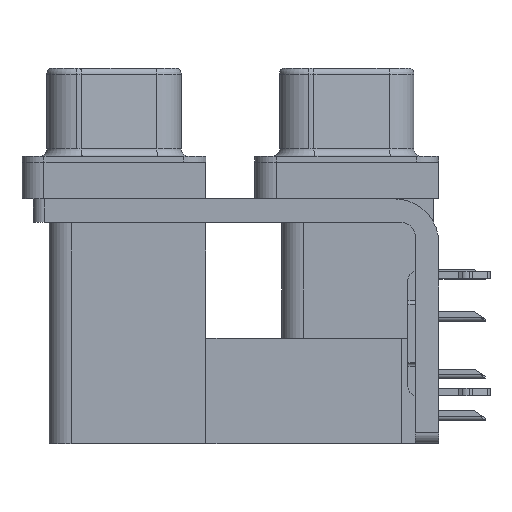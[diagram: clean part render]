
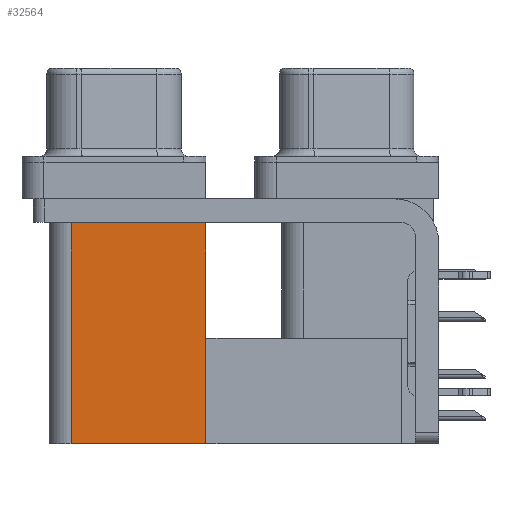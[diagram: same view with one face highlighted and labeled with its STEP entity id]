
A CAD part, left-side view. The second image highlights one B-rep face of the part: STEP entity #32564.
In plain terms, the highlighted planar face has unit normal (-1, 0, 0).
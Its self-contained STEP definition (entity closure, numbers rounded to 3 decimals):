
#817 = VERTEX_POINT ( 'NONE', #14173 ) ;
#1444 = DIRECTION ( 'NONE',  ( 1., 0., 0. ) ) ;
#4059 = CARTESIAN_POINT ( 'NONE',  ( 3.765, 9.6, -19.2 ) ) ;
#4253 = LINE ( 'NONE', #24593, #21638 ) ;
#4708 = CARTESIAN_POINT ( 'NONE',  ( 3.765, 9.6, -19.2 ) ) ;
#5044 = ORIENTED_EDGE ( 'NONE', *, *, #24231, .T. ) ;
#6314 = DIRECTION ( 'NONE',  ( 0., 1., 0. ) ) ;
#7275 = LINE ( 'NONE', #17641, #21232 ) ;
#7396 = DIRECTION ( 'NONE',  ( 0., 0., 1. ) ) ;
#7941 = VECTOR ( 'NONE', #7396, 1000. ) ;
#8353 = EDGE_CURVE ( 'NONE', #9491, #817, #4253, .T. ) ;
#9255 = CARTESIAN_POINT ( 'NONE',  ( 3.765, 18.8, -2.5 ) ) ;
#9491 = VERTEX_POINT ( 'NONE', #4059 ) ;
#9644 = CARTESIAN_POINT ( 'NONE',  ( 3.765, 9.6, -19.2 ) ) ;
#11456 = VERTEX_POINT ( 'NONE', #11956 ) ;
#11956 = CARTESIAN_POINT ( 'NONE',  ( 3.765, 9.6, -2.5 ) ) ;
#12588 = ORIENTED_EDGE ( 'NONE', *, *, #19171, .T. ) ;
#12897 = LINE ( 'NONE', #9644, #7941 ) ;
#12924 = VERTEX_POINT ( 'NONE', #9255 ) ;
#14031 = EDGE_LOOP ( 'NONE', ( #5044, #18680, #31664, #12588 ) ) ;
#14173 = CARTESIAN_POINT ( 'NONE',  ( 3.765, 18.8, -19.2 ) ) ;
#16333 = CARTESIAN_POINT ( 'NONE',  ( 3.765, 9.6, -2.5 ) ) ;
#17641 = CARTESIAN_POINT ( 'NONE',  ( 3.765, 18.8, -19.2 ) ) ;
#18680 = ORIENTED_EDGE ( 'NONE', *, *, #31631, .F. ) ;
#19171 = EDGE_CURVE ( 'NONE', #9491, #11456, #12897, .T. ) ;
#19914 = FACE_OUTER_BOUND ( 'NONE', #14031, .T. ) ;
#21163 = DIRECTION ( 'NONE',  ( 0., 1., 0. ) ) ;
#21232 = VECTOR ( 'NONE', #28128, 1000. ) ;
#21638 = VECTOR ( 'NONE', #6314, 1000. ) ;
#23458 = AXIS2_PLACEMENT_3D ( 'NONE', #4708, #1444, #25572 ) ;
#24231 = EDGE_CURVE ( 'NONE', #11456, #12924, #31800, .T. ) ;
#24593 = CARTESIAN_POINT ( 'NONE',  ( 3.765, 9.6, -19.2 ) ) ;
#25572 = DIRECTION ( 'NONE',  ( 0., 0., -1. ) ) ;
#27294 = VECTOR ( 'NONE', #21163, 1000. ) ;
#28128 = DIRECTION ( 'NONE',  ( 0., 0., 1. ) ) ;
#30374 = PLANE ( 'NONE',  #23458 ) ;
#31631 = EDGE_CURVE ( 'NONE', #817, #12924, #7275, .T. ) ;
#31664 = ORIENTED_EDGE ( 'NONE', *, *, #8353, .F. ) ;
#31800 = LINE ( 'NONE', #16333, #27294 ) ;
#32564 = ADVANCED_FACE ( 'NONE', ( #19914 ), #30374, .F. ) ;
